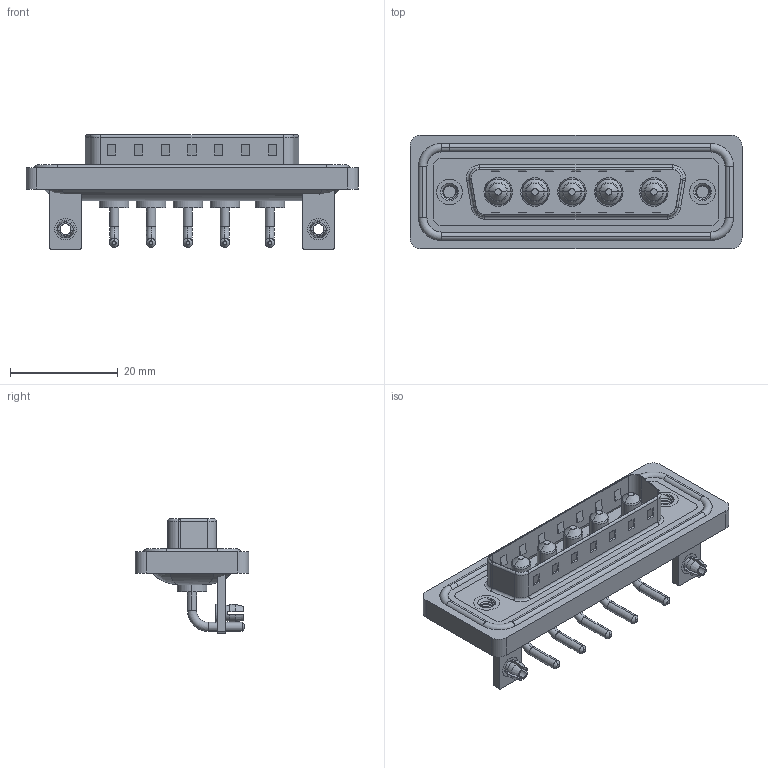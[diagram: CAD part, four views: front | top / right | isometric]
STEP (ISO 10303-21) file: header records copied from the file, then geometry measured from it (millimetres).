
FILE_DESCRIPTION (( 'STEP AP203' ), '1' );
FILE_NAME ('629W5W5-340-1N3.STEP', '2024-04-11T15:11:56', ( '' ), ( '' ), 'SwSTEP 2.0', 'SolidWorks 2023', '' );
FILE_SCHEMA (( 'CONFIG_CONTROL_DESIGN' ));
Length unit declared in the file: millimetre
Products named in the file (9): 629Combo Threaded Rivet_3; 629Combo Shell Front_25 Contacts; 629Combo Stabilizer Bracket; 629Combo Shell Rear_25 Contacts; 629Combo Waterproof Housing_25 Contacts; 629Combo Housing_5W5; 629Combo Board Lock; Power Pin_10A RA; 629W5W5-340-1N3
Assembly tree (15 placements, depth 2):
  629W5W5-340-1N3
    629Combo Housing_5W5
    629Combo Shell Rear_25 Contacts
    629Combo Shell Front_25 Contacts
    629Combo Waterproof Housing_25 Contacts
    629Combo Threaded Rivet_3  x2
    629Combo Stabilizer Bracket  x2
    629Combo Board Lock  x2
    Power Pin_10A RA  x5
Bounding box: 61.75 x 21.1 x 21.3 mm (x, y, z)
Volume: 7825.9 mm3; surface area: 12814.5 mm2
Topology: 21 solids, 21 shells, 830 faces, 2047 edges, 1291 vertices
Faces by surface type: cylinder 343, plane 327, torus 84, cone 61, bspline 15
Entity records: 20426 total; most frequent: CARTESIAN_POINT 4893, DIRECTION 3144, ORIENTED_EDGE 2930, EDGE_CURVE 1465, AXIS2_PLACEMENT_3D 1163, VERTEX_POINT 932, LINE 818, VECTOR 818
